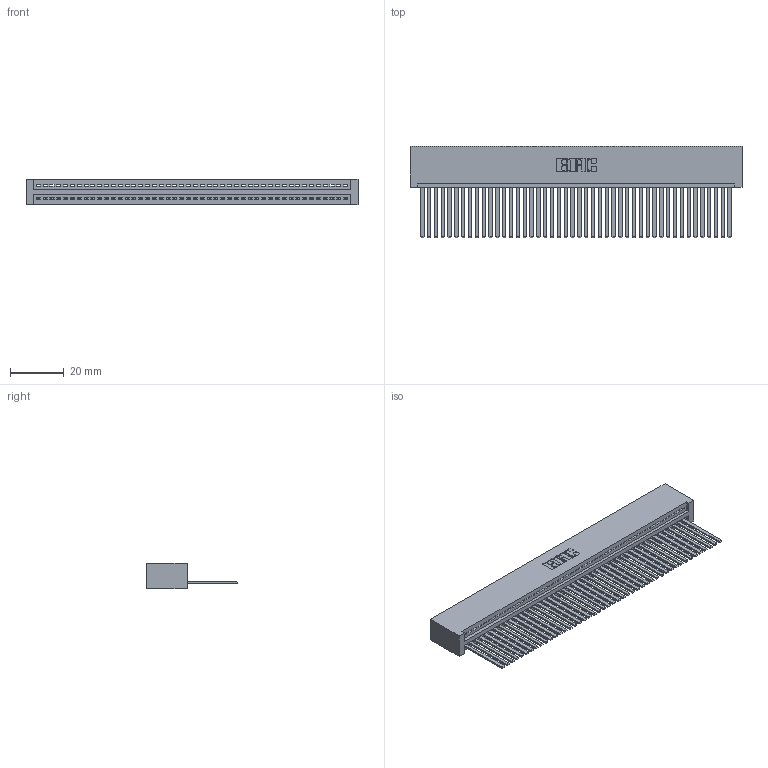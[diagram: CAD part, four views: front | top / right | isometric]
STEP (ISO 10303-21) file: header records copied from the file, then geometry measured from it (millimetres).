
FILE_DESCRIPTION (( 'STEP AP203' ), '1' );
FILE_NAME ('345-046-544-101.STEP', '2018-09-10T02:07:35', ( '' ), ( '' ), 'SwSTEP 2.0', 'SolidWorks 2016', '' );
FILE_SCHEMA (( 'CONFIG_CONTROL_DESIGN' ));
Length unit declared in the file: inch
Products named in the file (3): 345-292-001_345-293-144; 345-046-544-101; 345 Part_No Mounting Lugs
Assembly tree (47 placements, depth 2):
  345-046-544-101
    345 Part_No Mounting Lugs
    345-292-001_345-293-144  x46
Bounding box: 123.44 x 33.96 x 9.4 mm (x, y, z)
Volume: 12874.7 mm3; surface area: 18953.2 mm2
Topology: 47 solids, 47 shells, 2510 faces, 7585 edges, 4994 vertices
Faces by surface type: plane 1732, cylinder 778
Entity records: 33621 total; most frequent: CARTESIAN_POINT 5830, ORIENTED_EDGE 5810, DIRECTION 5077, EDGE_CURVE 2905, VECTOR 2601, LINE 2601, VERTEX_POINT 1934, AXIS2_PLACEMENT_3D 1238
